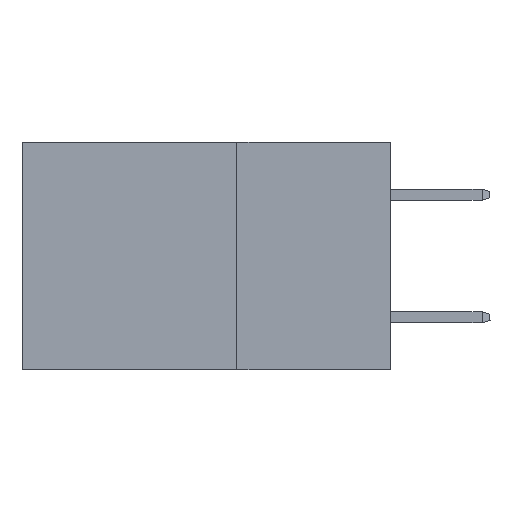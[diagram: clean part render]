
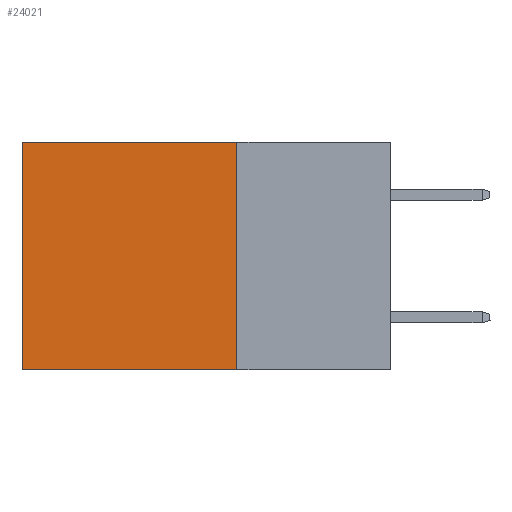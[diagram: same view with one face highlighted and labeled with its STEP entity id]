
A CAD part, left-side view. The second image highlights one B-rep face of the part: STEP entity #24021.
In plain terms, the highlighted planar face has unit normal (-1, 0, 0).
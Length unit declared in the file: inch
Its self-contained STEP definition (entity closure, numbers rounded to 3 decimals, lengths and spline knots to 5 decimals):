
#836 = DIRECTION ( 'NONE',  ( 0., 0., -1. ) ) ;
#1528 = LINE ( 'NONE', #11331, #21807 ) ;
#2158 = LINE ( 'NONE', #13453, #17047 ) ;
#3498 = ORIENTED_EDGE ( 'NONE', *, *, #18450, .F. ) ;
#6558 = DIRECTION ( 'NONE',  ( 0., 1., 0. ) ) ;
#7799 = ORIENTED_EDGE ( 'NONE', *, *, #16790, .F. ) ;
#7933 = VERTEX_POINT ( 'NONE', #19142 ) ;
#8877 = CARTESIAN_POINT ( 'NONE',  ( 0.2875, 0.25, 0. ) ) ;
#10817 = EDGE_CURVE ( 'NONE', #25582, #23591, #2158, .T. ) ;
#11331 = CARTESIAN_POINT ( 'NONE',  ( 0.2875, 0.25, 0. ) ) ;
#12402 = DIRECTION ( 'NONE',  ( 0., 1., 0. ) ) ;
#13041 = VECTOR ( 'NONE', #12402, 39.37008 ) ;
#13453 = CARTESIAN_POINT ( 'NONE',  ( 0.2875, 0.6, 0. ) ) ;
#13725 = CARTESIAN_POINT ( 'NONE',  ( 0.2875, 0.25, -0.37 ) ) ;
#14515 = CARTESIAN_POINT ( 'NONE',  ( 0.2875, 0.25, 0. ) ) ;
#15598 = ORIENTED_EDGE ( 'NONE', *, *, #10817, .T. ) ;
#16790 = EDGE_CURVE ( 'NONE', #7933, #23591, #22469, .T. ) ;
#17047 = VECTOR ( 'NONE', #836, 39.37008 ) ;
#17540 = AXIS2_PLACEMENT_3D ( 'NONE', #14515, #27352, #18429 ) ;
#18221 = EDGE_LOOP ( 'NONE', ( #15598, #7799, #3498, #27662 ) ) ;
#18429 = DIRECTION ( 'NONE',  ( 0., 0., -1. ) ) ;
#18450 = EDGE_CURVE ( 'NONE', #27980, #7933, #1528, .T. ) ;
#19142 = CARTESIAN_POINT ( 'NONE',  ( 0.2875, 0.25, -0.37 ) ) ;
#20006 = EDGE_CURVE ( 'NONE', #27980, #25582, #25770, .T. ) ;
#21486 = CARTESIAN_POINT ( 'NONE',  ( 0.2875, 0.6, -0.37 ) ) ;
#21807 = VECTOR ( 'NONE', #24224, 39.37008 ) ;
#21904 = CARTESIAN_POINT ( 'NONE',  ( 0.2875, 0.25, 0. ) ) ;
#22469 = LINE ( 'NONE', #13725, #13041 ) ;
#22878 = PLANE ( 'NONE',  #17540 ) ;
#23591 = VERTEX_POINT ( 'NONE', #21486 ) ;
#24021 = ADVANCED_FACE ( 'NONE', ( #26566 ), #22878, .F. ) ;
#24224 = DIRECTION ( 'NONE',  ( 0., 0., -1. ) ) ;
#25341 = CARTESIAN_POINT ( 'NONE',  ( 0.2875, 0.6, 0. ) ) ;
#25582 = VERTEX_POINT ( 'NONE', #25341 ) ;
#25770 = LINE ( 'NONE', #8877, #27491 ) ;
#26566 = FACE_OUTER_BOUND ( 'NONE', #18221, .T. ) ;
#27352 = DIRECTION ( 'NONE',  ( 1., 0., 0. ) ) ;
#27491 = VECTOR ( 'NONE', #6558, 39.37008 ) ;
#27662 = ORIENTED_EDGE ( 'NONE', *, *, #20006, .T. ) ;
#27980 = VERTEX_POINT ( 'NONE', #21904 ) ;
